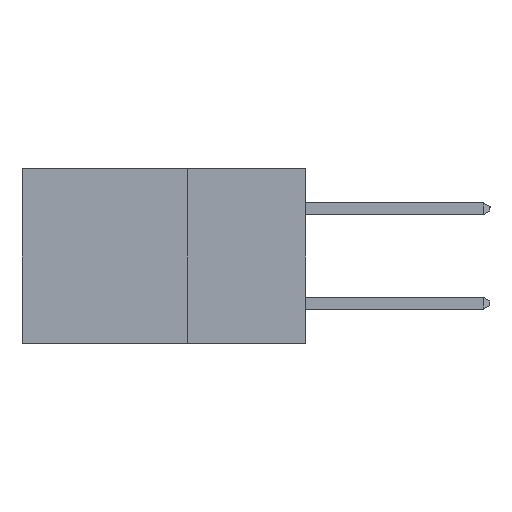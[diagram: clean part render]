
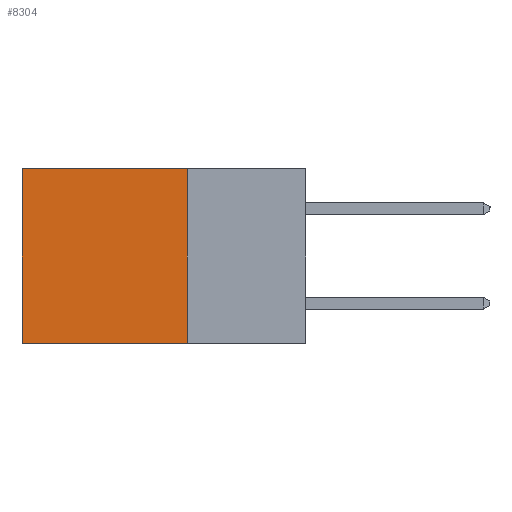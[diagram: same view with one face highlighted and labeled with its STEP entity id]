
A CAD part, left-side view. The second image highlights one B-rep face of the part: STEP entity #8304.
In plain terms, the highlighted planar face has unit normal (-1, 0, 0).
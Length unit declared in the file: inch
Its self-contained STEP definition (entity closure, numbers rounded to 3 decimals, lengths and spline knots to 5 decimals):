
#404 = PLANE ( 'NONE',  #9721 ) ;
#527 = VERTEX_POINT ( 'NONE', #8941 ) ;
#1936 = CARTESIAN_POINT ( 'NONE',  ( 0.2615, 0.25, 0. ) ) ;
#2767 = EDGE_CURVE ( 'NONE', #6417, #9945, #11865, .T. ) ;
#3025 = CARTESIAN_POINT ( 'NONE',  ( 0.2615, 0.6, 0. ) ) ;
#3478 = FACE_OUTER_BOUND ( 'NONE', #12343, .T. ) ;
#3567 = VECTOR ( 'NONE', #4453, 39.37008 ) ;
#4097 = ORIENTED_EDGE ( 'NONE', *, *, #8041, .T. ) ;
#4453 = DIRECTION ( 'NONE',  ( 0., 1., 0. ) ) ;
#5503 = CARTESIAN_POINT ( 'NONE',  ( 0.2615, 0.25, -0.37 ) ) ;
#5853 = ORIENTED_EDGE ( 'NONE', *, *, #12412, .F. ) ;
#5943 = CARTESIAN_POINT ( 'NONE',  ( 0.2615, 0.25, -0.37 ) ) ;
#6417 = VERTEX_POINT ( 'NONE', #12358 ) ;
#6465 = LINE ( 'NONE', #11580, #3567 ) ;
#6803 = DIRECTION ( 'NONE',  ( 0., 0., -1. ) ) ;
#7295 = DIRECTION ( 'NONE',  ( 0., 0., -1. ) ) ;
#7750 = VERTEX_POINT ( 'NONE', #3025 ) ;
#7772 = CARTESIAN_POINT ( 'NONE',  ( 0.2615, 0.6, -0.37 ) ) ;
#8041 = EDGE_CURVE ( 'NONE', #7750, #527, #11895, .T. ) ;
#8304 = ADVANCED_FACE ( 'NONE', ( #3478 ), #404, .F. ) ;
#8338 = DIRECTION ( 'NONE',  ( 0., 1., 0. ) ) ;
#8703 = DIRECTION ( 'NONE',  ( 0., 0., -1. ) ) ;
#8941 = CARTESIAN_POINT ( 'NONE',  ( 0.2615, 0.6, -0.37 ) ) ;
#9286 = VECTOR ( 'NONE', #8703, 39.37008 ) ;
#9721 = AXIS2_PLACEMENT_3D ( 'NONE', #5503, #11468, #7295 ) ;
#9945 = VERTEX_POINT ( 'NONE', #10212 ) ;
#10017 = EDGE_CURVE ( 'NONE', #6417, #7750, #11060, .T. ) ;
#10092 = ORIENTED_EDGE ( 'NONE', *, *, #10017, .T. ) ;
#10212 = CARTESIAN_POINT ( 'NONE',  ( 0.2615, 0.25, -0.37 ) ) ;
#10336 = VECTOR ( 'NONE', #8338, 39.37008 ) ;
#10663 = VECTOR ( 'NONE', #6803, 39.37008 ) ;
#11060 = LINE ( 'NONE', #1936, #10336 ) ;
#11165 = ORIENTED_EDGE ( 'NONE', *, *, #2767, .F. ) ;
#11468 = DIRECTION ( 'NONE',  ( 1., 0., 0. ) ) ;
#11580 = CARTESIAN_POINT ( 'NONE',  ( 0.2615, 0.25, -0.37 ) ) ;
#11865 = LINE ( 'NONE', #5943, #10663 ) ;
#11895 = LINE ( 'NONE', #7772, #9286 ) ;
#12343 = EDGE_LOOP ( 'NONE', ( #4097, #5853, #11165, #10092 ) ) ;
#12358 = CARTESIAN_POINT ( 'NONE',  ( 0.2615, 0.25, 0. ) ) ;
#12412 = EDGE_CURVE ( 'NONE', #9945, #527, #6465, .T. ) ;
